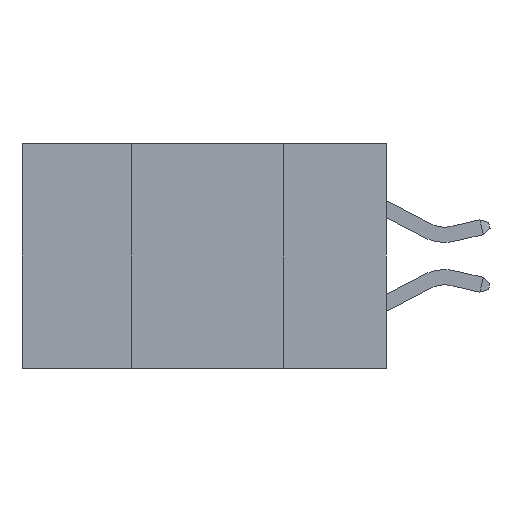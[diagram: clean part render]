
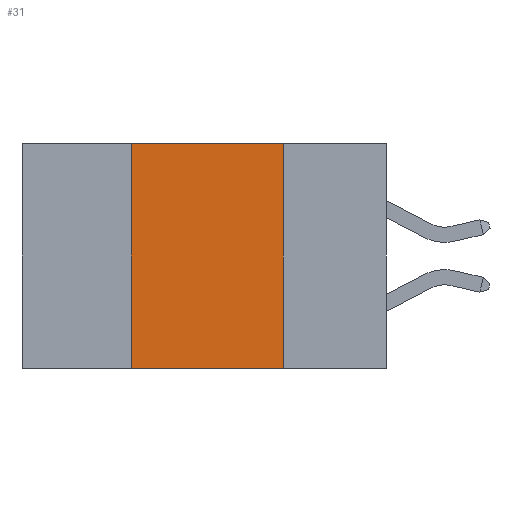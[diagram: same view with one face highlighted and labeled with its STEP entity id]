
A CAD part, left-side view. The second image highlights one B-rep face of the part: STEP entity #31.
In plain terms, the highlighted planar face has unit normal (-1, 0, 0).
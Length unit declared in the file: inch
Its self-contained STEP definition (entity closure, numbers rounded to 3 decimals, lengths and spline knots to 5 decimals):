
#31 = ADVANCED_FACE ( 'NONE', ( #125 ), #8102, .F. ) ;
#125 = FACE_OUTER_BOUND ( 'NONE', #3621, .T. ) ;
#767 = DIRECTION ( 'NONE',  ( 0., 0., -1. ) ) ;
#962 = EDGE_CURVE ( 'NONE', #5685, #7766, #2379, .T. ) ;
#1041 = ORIENTED_EDGE ( 'NONE', *, *, #3238, .F. ) ;
#1341 = CARTESIAN_POINT ( 'NONE',  ( 0., 0.6, -0.37 ) ) ;
#1729 = VECTOR ( 'NONE', #5407, 39.37008 ) ;
#2221 = CARTESIAN_POINT ( 'NONE',  ( 0., 0.17, 0. ) ) ;
#2379 = LINE ( 'NONE', #8604, #1729 ) ;
#2518 = DIRECTION ( 'NONE',  ( 0., 0., 1. ) ) ;
#2616 = CARTESIAN_POINT ( 'NONE',  ( 0., 0.42, -0.37 ) ) ;
#2986 = VECTOR ( 'NONE', #8025, 39.37008 ) ;
#3238 = EDGE_CURVE ( 'NONE', #10285, #5226, #4005, .T. ) ;
#3341 = CARTESIAN_POINT ( 'NONE',  ( 0., 0.6, 0. ) ) ;
#3621 = EDGE_LOOP ( 'NONE', ( #6809, #7562, #1041, #9233 ) ) ;
#4005 = LINE ( 'NONE', #9502, #7159 ) ;
#4008 = AXIS2_PLACEMENT_3D ( 'NONE', #3341, #7106, #767 ) ;
#4517 = DIRECTION ( 'NONE',  ( 0., -1., 0. ) ) ;
#5226 = VERTEX_POINT ( 'NONE', #10031 ) ;
#5407 = DIRECTION ( 'NONE',  ( 0., 0., -1. ) ) ;
#5685 = VERTEX_POINT ( 'NONE', #2221 ) ;
#5755 = CARTESIAN_POINT ( 'NONE',  ( 0., 0.6, 0. ) ) ;
#6507 = LINE ( 'NONE', #5755, #2986 ) ;
#6733 = CARTESIAN_POINT ( 'NONE',  ( 0., 0.17, -0.37 ) ) ;
#6809 = ORIENTED_EDGE ( 'NONE', *, *, #962, .F. ) ;
#6967 = VECTOR ( 'NONE', #4517, 39.37008 ) ;
#7106 = DIRECTION ( 'NONE',  ( 1., 0., 0. ) ) ;
#7159 = VECTOR ( 'NONE', #2518, 39.37008 ) ;
#7562 = ORIENTED_EDGE ( 'NONE', *, *, #9862, .F. ) ;
#7621 = LINE ( 'NONE', #1341, #6967 ) ;
#7766 = VERTEX_POINT ( 'NONE', #6733 ) ;
#7887 = EDGE_CURVE ( 'NONE', #10285, #7766, #7621, .T. ) ;
#8025 = DIRECTION ( 'NONE',  ( 0., -1., 0. ) ) ;
#8102 = PLANE ( 'NONE',  #4008 ) ;
#8604 = CARTESIAN_POINT ( 'NONE',  ( 0., 0.17, -0.37 ) ) ;
#9233 = ORIENTED_EDGE ( 'NONE', *, *, #7887, .T. ) ;
#9502 = CARTESIAN_POINT ( 'NONE',  ( 0., 0.42, -0.37 ) ) ;
#9862 = EDGE_CURVE ( 'NONE', #5226, #5685, #6507, .T. ) ;
#10031 = CARTESIAN_POINT ( 'NONE',  ( 0., 0.42, 0. ) ) ;
#10285 = VERTEX_POINT ( 'NONE', #2616 ) ;
